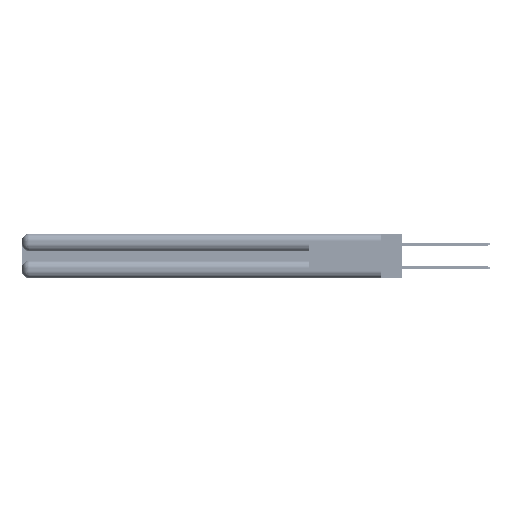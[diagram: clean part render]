
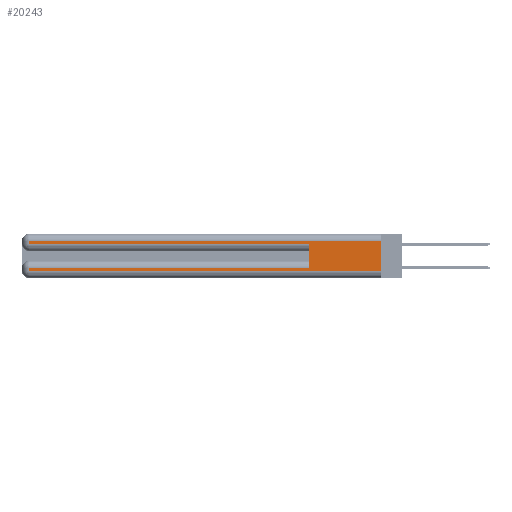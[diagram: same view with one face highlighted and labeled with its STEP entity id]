
A CAD part, left-side view. The second image highlights one B-rep face of the part: STEP entity #20243.
In plain terms, the highlighted planar face has unit normal (-1, 0, 0).
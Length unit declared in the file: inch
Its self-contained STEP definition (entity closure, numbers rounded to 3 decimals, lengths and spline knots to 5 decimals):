
#946 = CARTESIAN_POINT ( 'NONE',  ( 0., 2.94, 0.37 ) ) ;
#1158 = LINE ( 'NONE', #946, #46072 ) ;
#1774 = VECTOR ( 'NONE', #11303, 39.37008 ) ;
#1838 = LINE ( 'NONE', #4675, #35144 ) ;
#3194 = VECTOR ( 'NONE', #22966, 39.37008 ) ;
#4032 = VERTEX_POINT ( 'NONE', #17811 ) ;
#4675 = CARTESIAN_POINT ( 'NONE',  ( 0., 0., 0.37 ) ) ;
#5064 = EDGE_CURVE ( 'NONE', #43526, #16158, #36459, .T. ) ;
#7142 = CARTESIAN_POINT ( 'NONE',  ( 0., 0., 0.31 ) ) ;
#7608 = VERTEX_POINT ( 'NONE', #16828 ) ;
#7722 = EDGE_CURVE ( 'NONE', #18078, #7608, #43766, .T. ) ;
#7834 = EDGE_CURVE ( 'NONE', #22972, #4032, #38277, .T. ) ;
#8887 = ORIENTED_EDGE ( 'NONE', *, *, #27291, .F. ) ;
#8906 = EDGE_CURVE ( 'NONE', #16158, #22972, #18411, .T. ) ;
#9071 = DIRECTION ( 'NONE',  ( 0., 0., -1. ) ) ;
#9096 = CARTESIAN_POINT ( 'NONE',  ( 0., 2.94, 0.06 ) ) ;
#9833 = CARTESIAN_POINT ( 'NONE',  ( 0., 0.6, 0.145 ) ) ;
#10151 = CARTESIAN_POINT ( 'NONE',  ( 0., 2.94, 0.085 ) ) ;
#11303 = DIRECTION ( 'NONE',  ( 0., 1., 0. ) ) ;
#11960 = EDGE_CURVE ( 'NONE', #39275, #24055, #13401, .T. ) ;
#13401 = LINE ( 'NONE', #14650, #3194 ) ;
#13966 = DIRECTION ( 'NONE',  ( 0., -1., 0. ) ) ;
#14650 = CARTESIAN_POINT ( 'NONE',  ( 0., 0., 0.085 ) ) ;
#15143 = VECTOR ( 'NONE', #13966, 39.37008 ) ;
#15732 = CARTESIAN_POINT ( 'NONE',  ( 0., 2.94, 0.31 ) ) ;
#16158 = VERTEX_POINT ( 'NONE', #15732 ) ;
#16828 = CARTESIAN_POINT ( 'NONE',  ( 0., 0., 0.06 ) ) ;
#17811 = CARTESIAN_POINT ( 'NONE',  ( 0., 0.6, 0.285 ) ) ;
#18078 = VERTEX_POINT ( 'NONE', #9096 ) ;
#18411 = LINE ( 'NONE', #51689, #50402 ) ;
#18848 = ORIENTED_EDGE ( 'NONE', *, *, #7722, .T. ) ;
#20243 = ADVANCED_FACE ( 'NONE', ( #55776 ), #49156, .F. ) ;
#20556 = VECTOR ( 'NONE', #48011, 39.37008 ) ;
#22208 = CARTESIAN_POINT ( 'NONE',  ( 0., 0.6, 0.085 ) ) ;
#22966 = DIRECTION ( 'NONE',  ( 0., 1., 0. ) ) ;
#22972 = VERTEX_POINT ( 'NONE', #50732 ) ;
#23050 = DIRECTION ( 'NONE',  ( 0., 0., -1. ) ) ;
#24055 = VERTEX_POINT ( 'NONE', #10151 ) ;
#25223 = VECTOR ( 'NONE', #53345, 39.37008 ) ;
#26270 = ORIENTED_EDGE ( 'NONE', *, *, #7834, .T. ) ;
#27291 = EDGE_CURVE ( 'NONE', #43526, #7608, #1838, .T. ) ;
#27599 = CARTESIAN_POINT ( 'NONE',  ( 0., 0., 0.31 ) ) ;
#31749 = ORIENTED_EDGE ( 'NONE', *, *, #11960, .T. ) ;
#35144 = VECTOR ( 'NONE', #9071, 39.37008 ) ;
#36011 = DIRECTION ( 'NONE',  ( 1., 0., 0. ) ) ;
#36085 = EDGE_CURVE ( 'NONE', #39275, #4032, #38204, .T. ) ;
#36459 = LINE ( 'NONE', #7142, #1774 ) ;
#38204 = LINE ( 'NONE', #9833, #25223 ) ;
#38277 = LINE ( 'NONE', #39987, #15143 ) ;
#39275 = VERTEX_POINT ( 'NONE', #22208 ) ;
#39333 = EDGE_CURVE ( 'NONE', #24055, #18078, #1158, .T. ) ;
#39919 = DIRECTION ( 'NONE',  ( 0., 0., -1. ) ) ;
#39987 = CARTESIAN_POINT ( 'NONE',  ( 0., 0., 0.285 ) ) ;
#41948 = ORIENTED_EDGE ( 'NONE', *, *, #36085, .F. ) ;
#42982 = DIRECTION ( 'NONE',  ( 0., 0., -1. ) ) ;
#43526 = VERTEX_POINT ( 'NONE', #27599 ) ;
#43660 = CARTESIAN_POINT ( 'NONE',  ( 0., 0., 0.06 ) ) ;
#43766 = LINE ( 'NONE', #43660, #20556 ) ;
#44775 = CARTESIAN_POINT ( 'NONE',  ( 0., 0., 0.37 ) ) ;
#45397 = ORIENTED_EDGE ( 'NONE', *, *, #39333, .T. ) ;
#46072 = VECTOR ( 'NONE', #39919, 39.37008 ) ;
#46296 = ORIENTED_EDGE ( 'NONE', *, *, #5064, .T. ) ;
#48011 = DIRECTION ( 'NONE',  ( 0., -1., 0. ) ) ;
#49156 = PLANE ( 'NONE',  #55871 ) ;
#50402 = VECTOR ( 'NONE', #42982, 39.37008 ) ;
#50732 = CARTESIAN_POINT ( 'NONE',  ( 0., 2.94, 0.285 ) ) ;
#51689 = CARTESIAN_POINT ( 'NONE',  ( 0., 2.94, 0.37 ) ) ;
#52114 = EDGE_LOOP ( 'NONE', ( #8887, #46296, #52755, #26270, #41948, #31749, #45397, #18848 ) ) ;
#52755 = ORIENTED_EDGE ( 'NONE', *, *, #8906, .T. ) ;
#53345 = DIRECTION ( 'NONE',  ( 0., 0., 1. ) ) ;
#55776 = FACE_OUTER_BOUND ( 'NONE', #52114, .T. ) ;
#55871 = AXIS2_PLACEMENT_3D ( 'NONE', #44775, #36011, #23050 ) ;
